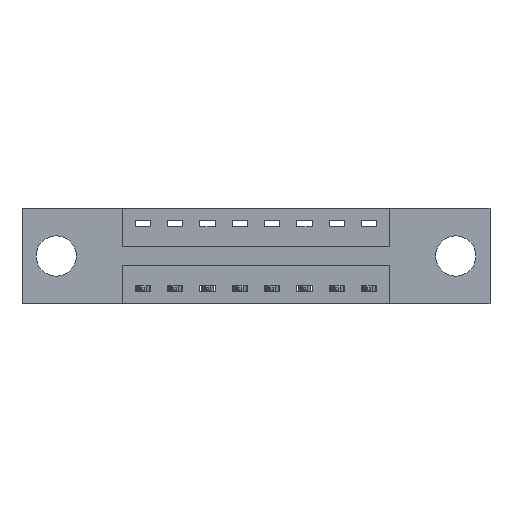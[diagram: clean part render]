
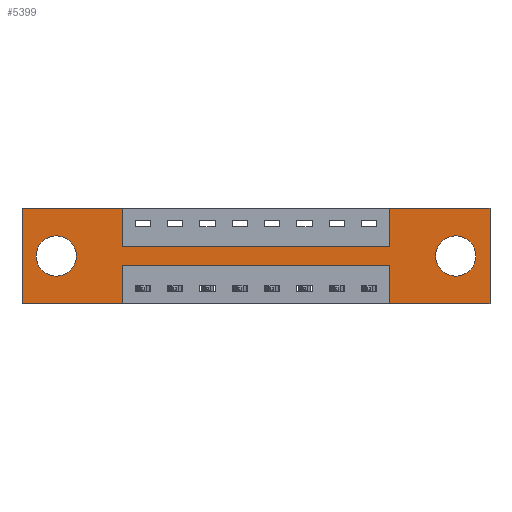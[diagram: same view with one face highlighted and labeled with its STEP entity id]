
A CAD part, front view. The second image highlights one B-rep face of the part: STEP entity #5399.
In plain terms, the highlighted planar face has unit normal (0, -1, 0).
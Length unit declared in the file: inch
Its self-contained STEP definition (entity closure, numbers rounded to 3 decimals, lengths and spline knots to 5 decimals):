
#129 = DIRECTION ( 'NONE',  ( 0., 0., -1. ) ) ;
#202 = DIRECTION ( 'NONE',  ( 0., 0., -1. ) ) ;
#364 = ORIENTED_EDGE ( 'NONE', *, *, #2305, .F. ) ;
#366 = AXIS2_PLACEMENT_3D ( 'NONE', #865, #6640, #1624 ) ;
#401 = CIRCLE ( 'NONE', #5410, 0.078 ) ;
#402 = VERTEX_POINT ( 'NONE', #2337 ) ;
#405 = ORIENTED_EDGE ( 'NONE', *, *, #8488, .F. ) ;
#436 = VECTOR ( 'NONE', #202, 39.37008 ) ;
#503 = CARTESIAN_POINT ( 'NONE',  ( 0., 0., -0.37 ) ) ;
#865 = CARTESIAN_POINT ( 'NONE',  ( 0.1325, 0., -0.185 ) ) ;
#1061 = CARTESIAN_POINT ( 'NONE',  ( 0., 0., 0. ) ) ;
#1180 = LINE ( 'NONE', #1355, #3714 ) ;
#1218 = DIRECTION ( 'NONE',  ( 0., 0., -1. ) ) ;
#1224 = DIRECTION ( 'NONE',  ( 0., 0., 1. ) ) ;
#1248 = VERTEX_POINT ( 'NONE', #3223 ) ;
#1260 = CARTESIAN_POINT ( 'NONE',  ( 0.1325, 0., -0.185 ) ) ;
#1263 = DIRECTION ( 'NONE',  ( 1., 0., 0. ) ) ;
#1355 = CARTESIAN_POINT ( 'NONE',  ( 0., 0., 0. ) ) ;
#1393 = LINE ( 'NONE', #6687, #3813 ) ;
#1454 = EDGE_CURVE ( 'NONE', #8946, #2074, #8196, .T. ) ;
#1470 = CARTESIAN_POINT ( 'NONE',  ( 1.4225, 0., -0.37 ) ) ;
#1624 = DIRECTION ( 'NONE',  ( 0., 0., 1. ) ) ;
#1682 = ORIENTED_EDGE ( 'NONE', *, *, #8047, .T. ) ;
#1834 = LINE ( 'NONE', #2055, #3552 ) ;
#1901 = VECTOR ( 'NONE', #1902, 39.37008 ) ;
#1902 = DIRECTION ( 'NONE',  ( -1., 0., 0. ) ) ;
#1939 = CARTESIAN_POINT ( 'NONE',  ( 1.6775, 0., -0.185 ) ) ;
#2036 = VECTOR ( 'NONE', #3262, 39.37008 ) ;
#2055 = CARTESIAN_POINT ( 'NONE',  ( 0.3875, 0., -0.22 ) ) ;
#2066 = ORIENTED_EDGE ( 'NONE', *, *, #6783, .F. ) ;
#2074 = VERTEX_POINT ( 'NONE', #1470 ) ;
#2084 = ORIENTED_EDGE ( 'NONE', *, *, #1454, .F. ) ;
#2085 = CARTESIAN_POINT ( 'NONE',  ( 0., 0., -0.37 ) ) ;
#2091 = AXIS2_PLACEMENT_3D ( 'NONE', #3412, #4092, #1218 ) ;
#2116 = LINE ( 'NONE', #2451, #6733 ) ;
#2267 = VERTEX_POINT ( 'NONE', #9100 ) ;
#2305 = EDGE_CURVE ( 'NONE', #4518, #8946, #6315, .T. ) ;
#2337 = CARTESIAN_POINT ( 'NONE',  ( 1.4225, 0., -0.15 ) ) ;
#2451 = CARTESIAN_POINT ( 'NONE',  ( 0.3875, 0., -0.15 ) ) ;
#2484 = VERTEX_POINT ( 'NONE', #4076 ) ;
#2499 = VERTEX_POINT ( 'NONE', #4040 ) ;
#2504 = CIRCLE ( 'NONE', #8673, 0.078 ) ;
#2603 = CARTESIAN_POINT ( 'NONE',  ( 0., 0., 0. ) ) ;
#2650 = CIRCLE ( 'NONE', #8155, 0.078 ) ;
#2683 = DIRECTION ( 'NONE',  ( 0., 1., 0. ) ) ;
#2699 = PLANE ( 'NONE',  #2091 ) ;
#2700 = VERTEX_POINT ( 'NONE', #7312 ) ;
#2871 = VERTEX_POINT ( 'NONE', #6763 ) ;
#2912 = EDGE_CURVE ( 'NONE', #2700, #8157, #4000, .T. ) ;
#2989 = EDGE_CURVE ( 'NONE', #2871, #8643, #5707, .T. ) ;
#3061 = CARTESIAN_POINT ( 'NONE',  ( 0.3875, 0., -0.37 ) ) ;
#3087 = ORIENTED_EDGE ( 'NONE', *, *, #7217, .F. ) ;
#3111 = EDGE_CURVE ( 'NONE', #2484, #1248, #2504, .T. ) ;
#3223 = CARTESIAN_POINT ( 'NONE',  ( 1.6775, 0., -0.107 ) ) ;
#3262 = DIRECTION ( 'NONE',  ( 0., 0., 1. ) ) ;
#3338 = EDGE_CURVE ( 'NONE', #4141, #2700, #1834, .T. ) ;
#3391 = CARTESIAN_POINT ( 'NONE',  ( 1.6775, 0., -0.185 ) ) ;
#3412 = CARTESIAN_POINT ( 'NONE',  ( 0., 0., -0.37 ) ) ;
#3552 = VECTOR ( 'NONE', #7210, 39.37008 ) ;
#3714 = VECTOR ( 'NONE', #1263, 39.37008 ) ;
#3755 = CARTESIAN_POINT ( 'NONE',  ( 1.81, 0., -0.37 ) ) ;
#3813 = VECTOR ( 'NONE', #8800, 39.37008 ) ;
#3850 = CARTESIAN_POINT ( 'NONE',  ( 1.81, 0., 0. ) ) ;
#4000 = LINE ( 'NONE', #3061, #8851 ) ;
#4040 = CARTESIAN_POINT ( 'NONE',  ( 0.3875, 0., -0.15 ) ) ;
#4076 = CARTESIAN_POINT ( 'NONE',  ( 1.6775, 0., -0.263 ) ) ;
#4092 = DIRECTION ( 'NONE',  ( 0., -1., 0. ) ) ;
#4133 = CARTESIAN_POINT ( 'NONE',  ( 0.3875, 0., -0.37 ) ) ;
#4141 = VERTEX_POINT ( 'NONE', #6610 ) ;
#4321 = LINE ( 'NONE', #8590, #5008 ) ;
#4324 = CARTESIAN_POINT ( 'NONE',  ( 1.81, 0., 0. ) ) ;
#4352 = CARTESIAN_POINT ( 'NONE',  ( 0.3875, 0., 0. ) ) ;
#4518 = VERTEX_POINT ( 'NONE', #4324 ) ;
#4752 = EDGE_LOOP ( 'NONE', ( #7322, #1682 ) ) ;
#4864 = DIRECTION ( 'NONE',  ( 0., 0., 1. ) ) ;
#4872 = EDGE_CURVE ( 'NONE', #2074, #4141, #4321, .T. ) ;
#4879 = EDGE_CURVE ( 'NONE', #1248, #2484, #401, .T. ) ;
#4906 = ORIENTED_EDGE ( 'NONE', *, *, #3338, .F. ) ;
#4932 = LINE ( 'NONE', #6664, #8280 ) ;
#5008 = VECTOR ( 'NONE', #4864, 39.37008 ) ;
#5076 = LINE ( 'NONE', #9105, #8766 ) ;
#5151 = ORIENTED_EDGE ( 'NONE', *, *, #5479, .F. ) ;
#5392 = DIRECTION ( 'NONE',  ( 1., 0., 0. ) ) ;
#5399 = ADVANCED_FACE ( 'NONE', ( #7775, #6851, #7425 ), #2699, .T. ) ;
#5410 = AXIS2_PLACEMENT_3D ( 'NONE', #1939, #2683, #7771 ) ;
#5479 = EDGE_CURVE ( 'NONE', #8157, #2871, #7885, .T. ) ;
#5542 = VECTOR ( 'NONE', #9409, 39.37008 ) ;
#5637 = ORIENTED_EDGE ( 'NONE', *, *, #4872, .F. ) ;
#5707 = LINE ( 'NONE', #1061, #2036 ) ;
#5710 = ORIENTED_EDGE ( 'NONE', *, *, #2989, .F. ) ;
#6067 = DIRECTION ( 'NONE',  ( 0., 0., 1. ) ) ;
#6276 = DIRECTION ( 'NONE',  ( 0., 1., 0. ) ) ;
#6315 = LINE ( 'NONE', #3850, #436 ) ;
#6372 = EDGE_CURVE ( 'NONE', #9004, #2267, #7517, .T. ) ;
#6528 = EDGE_LOOP ( 'NONE', ( #6936, #4906, #5637, #2084, #364, #3087, #9429, #405, #8031, #2066, #5710, #5151 ) ) ;
#6610 = CARTESIAN_POINT ( 'NONE',  ( 1.4225, 0., -0.22 ) ) ;
#6629 = ORIENTED_EDGE ( 'NONE', *, *, #3111, .T. ) ;
#6640 = DIRECTION ( 'NONE',  ( 0., 1., 0. ) ) ;
#6664 = CARTESIAN_POINT ( 'NONE',  ( 0.3875, 0., 0. ) ) ;
#6687 = CARTESIAN_POINT ( 'NONE',  ( 0., 0., 0. ) ) ;
#6733 = VECTOR ( 'NONE', #5392, 39.37008 ) ;
#6763 = CARTESIAN_POINT ( 'NONE',  ( 0., 0., -0.37 ) ) ;
#6783 = EDGE_CURVE ( 'NONE', #8643, #9564, #1180, .T. ) ;
#6851 = FACE_BOUND ( 'NONE', #4752, .T. ) ;
#6926 = ORIENTED_EDGE ( 'NONE', *, *, #4879, .T. ) ;
#6936 = ORIENTED_EDGE ( 'NONE', *, *, #2912, .F. ) ;
#7065 = EDGE_CURVE ( 'NONE', #402, #7118, #5076, .T. ) ;
#7118 = VERTEX_POINT ( 'NONE', #8510 ) ;
#7210 = DIRECTION ( 'NONE',  ( -1., 0., 0. ) ) ;
#7217 = EDGE_CURVE ( 'NONE', #7118, #4518, #1393, .T. ) ;
#7312 = CARTESIAN_POINT ( 'NONE',  ( 0.3875, 0., -0.22 ) ) ;
#7322 = ORIENTED_EDGE ( 'NONE', *, *, #6372, .T. ) ;
#7377 = DIRECTION ( 'NONE',  ( 0., 0., -1. ) ) ;
#7425 = FACE_OUTER_BOUND ( 'NONE', #6528, .T. ) ;
#7517 = CIRCLE ( 'NONE', #366, 0.078 ) ;
#7771 = DIRECTION ( 'NONE',  ( 0., 0., -1. ) ) ;
#7775 = FACE_BOUND ( 'NONE', #9377, .T. ) ;
#7885 = LINE ( 'NONE', #503, #1901 ) ;
#8031 = ORIENTED_EDGE ( 'NONE', *, *, #8327, .F. ) ;
#8047 = EDGE_CURVE ( 'NONE', #2267, #9004, #2650, .T. ) ;
#8155 = AXIS2_PLACEMENT_3D ( 'NONE', #1260, #9289, #1224 ) ;
#8157 = VERTEX_POINT ( 'NONE', #4133 ) ;
#8196 = LINE ( 'NONE', #2085, #5542 ) ;
#8280 = VECTOR ( 'NONE', #7377, 39.37008 ) ;
#8327 = EDGE_CURVE ( 'NONE', #9564, #2499, #4932, .T. ) ;
#8488 = EDGE_CURVE ( 'NONE', #2499, #402, #2116, .T. ) ;
#8510 = CARTESIAN_POINT ( 'NONE',  ( 1.4225, 0., 0. ) ) ;
#8590 = CARTESIAN_POINT ( 'NONE',  ( 1.4225, 0., -0.37 ) ) ;
#8643 = VERTEX_POINT ( 'NONE', #2603 ) ;
#8673 = AXIS2_PLACEMENT_3D ( 'NONE', #3391, #6276, #9284 ) ;
#8766 = VECTOR ( 'NONE', #6067, 39.37008 ) ;
#8800 = DIRECTION ( 'NONE',  ( 1., 0., 0. ) ) ;
#8851 = VECTOR ( 'NONE', #129, 39.37008 ) ;
#8946 = VERTEX_POINT ( 'NONE', #3755 ) ;
#8970 = CARTESIAN_POINT ( 'NONE',  ( 0.1325, 0., -0.107 ) ) ;
#9004 = VERTEX_POINT ( 'NONE', #8970 ) ;
#9100 = CARTESIAN_POINT ( 'NONE',  ( 0.1325, 0., -0.263 ) ) ;
#9105 = CARTESIAN_POINT ( 'NONE',  ( 1.4225, 0., 0. ) ) ;
#9284 = DIRECTION ( 'NONE',  ( 0., 0., -1. ) ) ;
#9289 = DIRECTION ( 'NONE',  ( 0., 1., 0. ) ) ;
#9377 = EDGE_LOOP ( 'NONE', ( #6926, #6629 ) ) ;
#9409 = DIRECTION ( 'NONE',  ( -1., 0., 0. ) ) ;
#9429 = ORIENTED_EDGE ( 'NONE', *, *, #7065, .F. ) ;
#9564 = VERTEX_POINT ( 'NONE', #4352 ) ;
